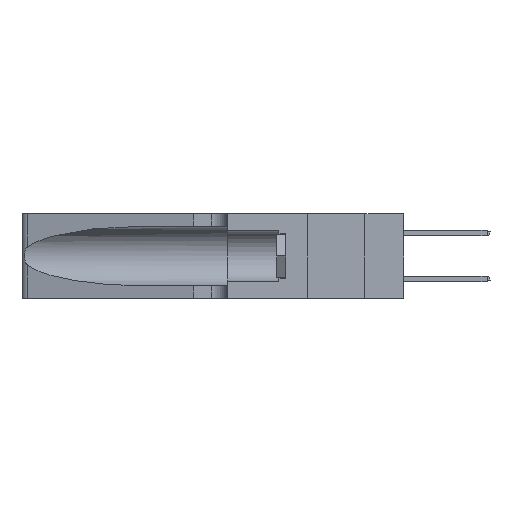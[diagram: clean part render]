
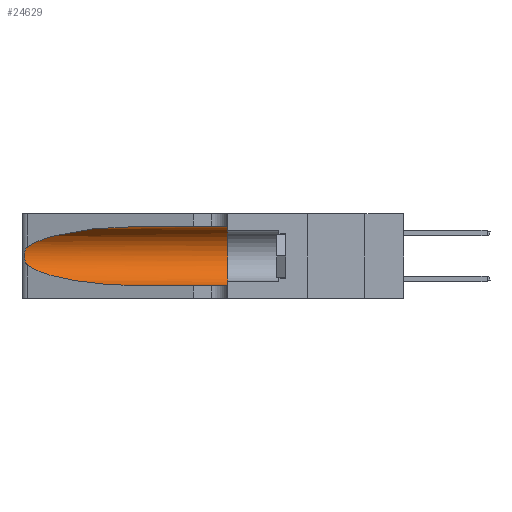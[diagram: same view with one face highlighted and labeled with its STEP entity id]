
A CAD part, left-side view. The second image highlights one B-rep face of the part: STEP entity #24629.
In plain terms, the highlighted cylindrical face has radius 3.308 mm (diameter 6.617 mm), a partial arc.
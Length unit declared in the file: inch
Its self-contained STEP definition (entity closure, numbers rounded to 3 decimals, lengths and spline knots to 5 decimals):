
#857 = ORIENTED_EDGE ( 'NONE', *, *, #6851, .T. ) ;
#1945 = CARTESIAN_POINT ( 'NONE',  ( 0.1305, 1.61858, 0.05475 ) ) ;
#2635 = CARTESIAN_POINT ( 'NONE',  ( 0.1305, 0.35, 0.185 ) ) ;
#3028 = LINE ( 'NONE', #1945, #31696 ) ;
#3137 = EDGE_CURVE ( 'NONE', #42599, #10618, #42609, .T. ) ;
#4707 = FACE_OUTER_BOUND ( 'NONE', #14524, .T. ) ;
#5091 = CARTESIAN_POINT ( 'NONE',  ( 0.1305, 0.35, 0.31525 ) ) ;
#6200 = VERTEX_POINT ( 'NONE', #7084 ) ;
#6816 = CARTESIAN_POINT ( 'NONE',  ( 0.26018, 1.23835, 0.19895 ) ) ;
#6851 = EDGE_CURVE ( 'NONE', #6200, #19410, #43478, .T. ) ;
#7084 = CARTESIAN_POINT ( 'NONE',  ( 0.1305, 0.72297, 0.31525 ) ) ;
#8638 = ORIENTED_EDGE ( 'NONE', *, *, #21632, .F. ) ;
#10376 = AXIS2_PLACEMENT_3D ( 'NONE', #2635, #13290, #39669 ) ;
#10442 = LINE ( 'NONE', #44707, #14544 ) ;
#10618 = VERTEX_POINT ( 'NONE', #31803 ) ;
#12329 = CYLINDRICAL_SURFACE ( 'NONE', #38287, 0.13025 ) ;
#13062 = ORIENTED_EDGE ( 'NONE', *, *, #23896, .T. ) ;
#13153 = CARTESIAN_POINT ( 'NONE',  ( 0.1305, 1.61858, 0.185 ) ) ;
#13290 = DIRECTION ( 'NONE',  ( 0., 1., 0. ) ) ;
#13677 = CARTESIAN_POINT ( 'NONE',  ( 0.25555, 1.22993, 0.14849 ) ) ;
#13840 = CARTESIAN_POINT ( 'NONE',  ( 0.26075, 1.23896, 0.19203 ) ) ;
#14524 = EDGE_LOOP ( 'NONE', ( #857, #36591, #46344, #13062, #8638, #18876 ) ) ;
#14544 = VECTOR ( 'NONE', #26301, 39.37008 ) ;
#17442 = CARTESIAN_POINT ( 'NONE',  ( 0.25555, 1.22994, 0.2215 ) ) ;
#18876 = ORIENTED_EDGE ( 'NONE', *, *, #34029, .F. ) ;
#19410 = VERTEX_POINT ( 'NONE', #38994 ) ;
#20042 = CARTESIAN_POINT ( 'NONE',  ( 0.18966, 0.96281, 0.31525 ) ) ;
#20712 = CARTESIAN_POINT ( 'NONE',  ( 0.1305, 0.35, 0.05475 ) ) ;
#21199 = CARTESIAN_POINT ( 'NONE',  ( 0.25639, 1.23186, 0.15144 ) ) ;
#21509 = CARTESIAN_POINT ( 'NONE',  ( 0.25639, 1.23184, 0.21858 ) ) ;
#21632 = EDGE_CURVE ( 'NONE', #45363, #28433, #23215, .T. ) ;
#22120 = CARTESIAN_POINT ( 'NONE',  ( 0.18966, 0.96281, 0.05475 ) ) ;
#23215 = CIRCLE ( 'NONE', #10376, 0.13025 ) ;
#23896 = EDGE_CURVE ( 'NONE', #10618, #28433, #3028, .T. ) ;
#24149 = CARTESIAN_POINT ( 'NONE',  ( 0.1305, 0.72297, 0.31525 ) ) ;
#24629 = ADVANCED_FACE ( 'NONE', ( #4707 ), #12329, .F. ) ;
#25439 = CARTESIAN_POINT ( 'NONE',  ( 0.25854, 1.2359, 0.20912 ) ) ;
#25594 = CARTESIAN_POINT ( 'NONE',  ( 0.26075, 1.23896, 0.178 ) ) ;
#26301 = DIRECTION ( 'NONE',  ( 0., -1., 0. ) ) ;
#27908 = CARTESIAN_POINT ( 'NONE',  ( 0.2373, 1.15595, 0.28018 ) ) ;
#28433 = VERTEX_POINT ( 'NONE', #20712 ) ;
#29633 = CARTESIAN_POINT ( 'NONE',  ( 0.1305, 0.72297, 0.05475 ) ) ;
#31696 = VECTOR ( 'NONE', #43186, 39.37008 ) ;
#31803 = CARTESIAN_POINT ( 'NONE',  ( 0.1305, 0.72297, 0.05475 ) ) ;
#32294 = CARTESIAN_POINT ( 'NONE',  ( 0.25789, 1.23486, 0.15765 ) ) ;
#32903 = CARTESIAN_POINT ( 'NONE',  ( 0.25487, 1.22718, 0.14631 ) ) ;
#34029 = EDGE_CURVE ( 'NONE', #6200, #45363, #10442, .T. ) ;
#34834 = B_SPLINE_CURVE_WITH_KNOTS ( 'NONE', 3,
 ( #47730, #17442, #21509, #36322, #25439, #6816, #13840, #25594, #40214, #43487, #32294, #21199, #13677, #47258 ),
 .UNSPECIFIED., .F., .F.,
 ( 4, 2, 2, 2, 2, 2, 4 ),
 ( 0., 0.00027, 0.00053, 0.00107, 0.0016, 0.00187, 0.00214 ),
 .UNSPECIFIED. ) ;
#35963 = DIRECTION ( 'NONE',  ( 0., -1., 0. ) ) ;
#36322 = CARTESIAN_POINT ( 'NONE',  ( 0.25787, 1.23484, 0.2124 ) ) ;
#36591 = ORIENTED_EDGE ( 'NONE', *, *, #47909, .T. ) ;
#38287 = AXIS2_PLACEMENT_3D ( 'NONE', #13153, #35963, #42976 ) ;
#38994 = CARTESIAN_POINT ( 'NONE',  ( 0.25487, 1.22718, 0.22369 ) ) ;
#39669 = DIRECTION ( 'NONE',  ( 0., 0., 1. ) ) ;
#40214 = CARTESIAN_POINT ( 'NONE',  ( 0.26017, 1.23833, 0.17102 ) ) ;
#42599 = VERTEX_POINT ( 'NONE', #32903 ) ;
#42609 =( BOUNDED_CURVE ( )  B_SPLINE_CURVE ( 3, ( #44256, #48013, #22120, #29633 ),
 .UNSPECIFIED., .F., .F. ) 
 B_SPLINE_CURVE_WITH_KNOTS ( ( 4, 4 ),
 ( 3.44316, 4.71239 ),
 .UNSPECIFIED. ) 
 CURVE ( )  GEOMETRIC_REPRESENTATION_ITEM ( )  RATIONAL_B_SPLINE_CURVE ( ( 1., 0.87, 0.87, 1. ) ) 
 REPRESENTATION_ITEM ( '' )  );
#42976 = DIRECTION ( 'NONE',  ( 0., 0., -1. ) ) ;
#43186 = DIRECTION ( 'NONE',  ( 0., -1., 0. ) ) ;
#43478 =( BOUNDED_CURVE ( )  B_SPLINE_CURVE ( 3, ( #24149, #20042, #27908, #46134 ),
 .UNSPECIFIED., .F., .F. ) 
 B_SPLINE_CURVE_WITH_KNOTS ( ( 4, 4 ),
 ( 1.5708, 2.84003 ),
 .UNSPECIFIED. ) 
 CURVE ( )  GEOMETRIC_REPRESENTATION_ITEM ( )  RATIONAL_B_SPLINE_CURVE ( ( 1., 0.87, 0.87, 1. ) ) 
 REPRESENTATION_ITEM ( '' )  );
#43487 = CARTESIAN_POINT ( 'NONE',  ( 0.25856, 1.23593, 0.16098 ) ) ;
#44256 = CARTESIAN_POINT ( 'NONE',  ( 0.25487, 1.22718, 0.14631 ) ) ;
#44707 = CARTESIAN_POINT ( 'NONE',  ( 0.1305, 1.61858, 0.31525 ) ) ;
#45363 = VERTEX_POINT ( 'NONE', #5091 ) ;
#46134 = CARTESIAN_POINT ( 'NONE',  ( 0.25487, 1.22718, 0.22369 ) ) ;
#46344 = ORIENTED_EDGE ( 'NONE', *, *, #3137, .T. ) ;
#47258 = CARTESIAN_POINT ( 'NONE',  ( 0.25487, 1.22718, 0.14631 ) ) ;
#47730 = CARTESIAN_POINT ( 'NONE',  ( 0.25487, 1.22718, 0.22369 ) ) ;
#47909 = EDGE_CURVE ( 'NONE', #19410, #42599, #34834, .T. ) ;
#48013 = CARTESIAN_POINT ( 'NONE',  ( 0.2373, 1.15595, 0.08982 ) ) ;
